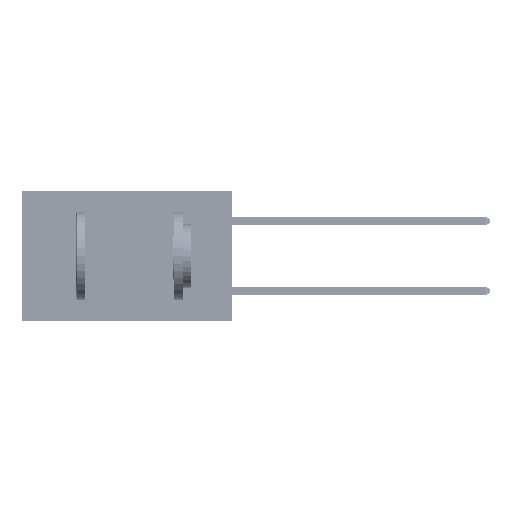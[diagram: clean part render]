
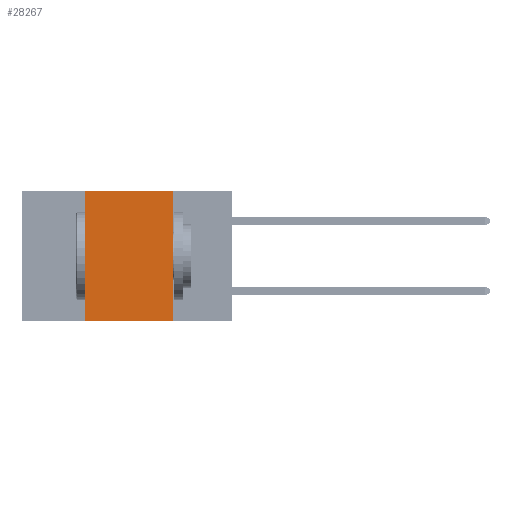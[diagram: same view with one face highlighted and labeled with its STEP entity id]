
A CAD part, left-side view. The second image highlights one B-rep face of the part: STEP entity #28267.
In plain terms, the highlighted planar face has unit normal (-1, 0, 0).
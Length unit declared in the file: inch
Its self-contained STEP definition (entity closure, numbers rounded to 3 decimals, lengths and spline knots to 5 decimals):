
#1275 = EDGE_CURVE ( 'NONE', #44524, #15132, #31350, .T. ) ;
#1305 = EDGE_LOOP ( 'NONE', ( #20322, #44597, #24398, #15980 ) ) ;
#2385 = DIRECTION ( 'NONE',  ( 1., 0., 0. ) ) ;
#2912 = PLANE ( 'NONE',  #42995 ) ;
#3041 = VECTOR ( 'NONE', #42018, 39.37008 ) ;
#4657 = FACE_OUTER_BOUND ( 'NONE', #1305, .T. ) ;
#5770 = CARTESIAN_POINT ( 'NONE',  ( 0., 0.42, 0. ) ) ;
#6995 = CARTESIAN_POINT ( 'NONE',  ( 0., 0.6, 0. ) ) ;
#7277 = EDGE_CURVE ( 'NONE', #15132, #50864, #30617, .T. ) ;
#12455 = DIRECTION ( 'NONE',  ( 0., -1., 0. ) ) ;
#12631 = VERTEX_POINT ( 'NONE', #30266 ) ;
#15132 = VERTEX_POINT ( 'NONE', #29160 ) ;
#15727 = CARTESIAN_POINT ( 'NONE',  ( 0., 0.17, 0. ) ) ;
#15980 = ORIENTED_EDGE ( 'NONE', *, *, #29662, .T. ) ;
#16147 = DIRECTION ( 'NONE',  ( 0., -1., 0. ) ) ;
#16659 = CARTESIAN_POINT ( 'NONE',  ( 0., 0.6, 0. ) ) ;
#19170 = EDGE_CURVE ( 'NONE', #12631, #44524, #25169, .T. ) ;
#20322 = ORIENTED_EDGE ( 'NONE', *, *, #7277, .F. ) ;
#20460 = CARTESIAN_POINT ( 'NONE',  ( 0., 0.42, 0. ) ) ;
#22406 = VECTOR ( 'NONE', #12455, 39.37008 ) ;
#24398 = ORIENTED_EDGE ( 'NONE', *, *, #19170, .F. ) ;
#24743 = VECTOR ( 'NONE', #16147, 39.37008 ) ;
#25169 = LINE ( 'NONE', #5770, #3041 ) ;
#26100 = CARTESIAN_POINT ( 'NONE',  ( 0., 0.17, -0.37 ) ) ;
#28267 = ADVANCED_FACE ( 'NONE', ( #4657 ), #2912, .F. ) ;
#29160 = CARTESIAN_POINT ( 'NONE',  ( 0., 0.17, 0. ) ) ;
#29662 = EDGE_CURVE ( 'NONE', #12631, #50864, #48834, .T. ) ;
#30266 = CARTESIAN_POINT ( 'NONE',  ( 0., 0.42, -0.37 ) ) ;
#30617 = LINE ( 'NONE', #15727, #40081 ) ;
#31350 = LINE ( 'NONE', #16659, #22406 ) ;
#36124 = CARTESIAN_POINT ( 'NONE',  ( 0., 0.6, -0.37 ) ) ;
#36238 = DIRECTION ( 'NONE',  ( 0., 0., -1. ) ) ;
#40081 = VECTOR ( 'NONE', #36238, 39.37008 ) ;
#42018 = DIRECTION ( 'NONE',  ( 0., 0., 1. ) ) ;
#42995 = AXIS2_PLACEMENT_3D ( 'NONE', #6995, #2385, #43415 ) ;
#43415 = DIRECTION ( 'NONE',  ( 0., 0., -1. ) ) ;
#44524 = VERTEX_POINT ( 'NONE', #20460 ) ;
#44597 = ORIENTED_EDGE ( 'NONE', *, *, #1275, .F. ) ;
#48834 = LINE ( 'NONE', #36124, #24743 ) ;
#50864 = VERTEX_POINT ( 'NONE', #26100 ) ;
